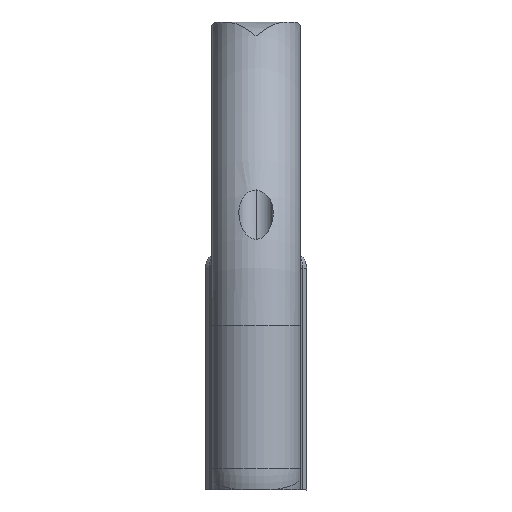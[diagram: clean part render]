
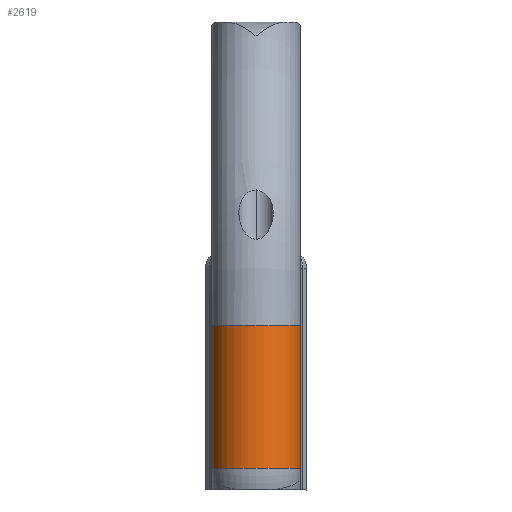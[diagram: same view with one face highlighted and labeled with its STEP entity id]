
A CAD part, front view. The second image highlights one B-rep face of the part: STEP entity #2619.
In plain terms, the highlighted cylindrical face has radius 11.509 mm (diameter 23.019 mm), a partial arc.
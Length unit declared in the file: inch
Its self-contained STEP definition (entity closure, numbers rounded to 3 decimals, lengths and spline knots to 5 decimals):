
#283 = VECTOR ( 'NONE', #3958, 39.37008 ) ;
#296 = LINE ( 'NONE', #3926, #283 ) ;
#452 = AXIS2_PLACEMENT_3D ( 'NONE', #3614, #3589, #3536 ) ;
#466 = CARTESIAN_POINT ( 'NONE',  ( 5.42884, 2.82407, 8.02732 ) ) ;
#509 = CIRCLE ( 'NONE', #2643, 0.45312 ) ;
#610 = ORIENTED_EDGE ( 'NONE', *, *, #3464, .F. ) ;
#1120 = DIRECTION ( 'NONE',  ( 0., 1., 0. ) ) ;
#1162 = DIRECTION ( 'NONE',  ( 0., 0., 1. ) ) ;
#1179 = CARTESIAN_POINT ( 'NONE',  ( 4.97571, 2.82407, 8.02732 ) ) ;
#1199 = AXIS2_PLACEMENT_3D ( 'NONE', #1179, #1162, #1120 ) ;
#1336 = ORIENTED_EDGE ( 'NONE', *, *, #4247, .F. ) ;
#1348 = ORIENTED_EDGE ( 'NONE', *, *, #2239, .F. ) ;
#1499 = ORIENTED_EDGE ( 'NONE', *, *, #3243, .T. ) ;
#1726 = CARTESIAN_POINT ( 'NONE',  ( 5.42884, 2.82407, 6.56902 ) ) ;
#1806 = DIRECTION ( 'NONE',  ( 0., 0., 1. ) ) ;
#1817 = CARTESIAN_POINT ( 'NONE',  ( 4.52259, 2.82407, 6.56902 ) ) ;
#1830 = CARTESIAN_POINT ( 'NONE',  ( 4.52259, 2.82407, 8.02732 ) ) ;
#1980 = EDGE_LOOP ( 'NONE', ( #1348, #1336, #1499, #610 ) ) ;
#2106 = CARTESIAN_POINT ( 'NONE',  ( 4.52259, 2.82407, 8.02732 ) ) ;
#2122 = VERTEX_POINT ( 'NONE', #1726 ) ;
#2239 = EDGE_CURVE ( 'NONE', #3369, #3752, #2276, .T. ) ;
#2276 = CIRCLE ( 'NONE', #1199, 0.45313 ) ;
#2619 = ADVANCED_FACE ( 'NONE', ( #3834 ), #3783, .T. ) ;
#2643 = AXIS2_PLACEMENT_3D ( 'NONE', #3909, #3913, #3899 ) ;
#3243 = EDGE_CURVE ( 'NONE', #3583, #2122, #509, .T. ) ;
#3369 = VERTEX_POINT ( 'NONE', #2106 ) ;
#3464 = EDGE_CURVE ( 'NONE', #3752, #2122, #296, .T. ) ;
#3536 = DIRECTION ( 'NONE',  ( 1., 0., 0. ) ) ;
#3583 = VERTEX_POINT ( 'NONE', #1817 ) ;
#3589 = DIRECTION ( 'NONE',  ( 0., 0., 1. ) ) ;
#3614 = CARTESIAN_POINT ( 'NONE',  ( 4.97571, 2.82407, 8.02732 ) ) ;
#3752 = VERTEX_POINT ( 'NONE', #466 ) ;
#3783 = CYLINDRICAL_SURFACE ( 'NONE', #452, 0.45312 ) ;
#3834 = FACE_OUTER_BOUND ( 'NONE', #1980, .T. ) ;
#3899 = DIRECTION ( 'NONE',  ( 1., 0., 0. ) ) ;
#3909 = CARTESIAN_POINT ( 'NONE',  ( 4.97571, 2.82407, 6.56902 ) ) ;
#3913 = DIRECTION ( 'NONE',  ( 0., 0., 1. ) ) ;
#3926 = CARTESIAN_POINT ( 'NONE',  ( 5.42884, 2.82407, 11.88889 ) ) ;
#3958 = DIRECTION ( 'NONE',  ( 0., 0., -1. ) ) ;
#4149 = VECTOR ( 'NONE', #1806, 39.37008 ) ;
#4169 = LINE ( 'NONE', #1830, #4149 ) ;
#4247 = EDGE_CURVE ( 'NONE', #3583, #3369, #4169, .T. ) ;
